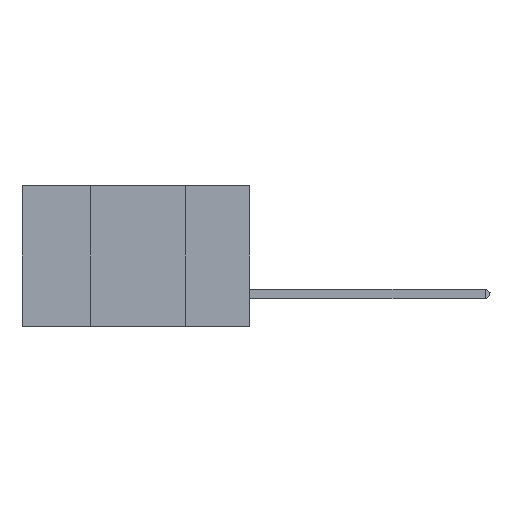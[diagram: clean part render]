
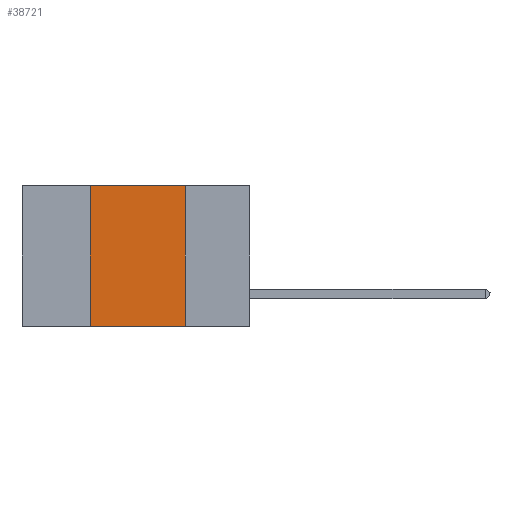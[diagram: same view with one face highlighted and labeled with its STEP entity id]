
A CAD part, left-side view. The second image highlights one B-rep face of the part: STEP entity #38721.
In plain terms, the highlighted planar face has unit normal (-1, 0, 0).
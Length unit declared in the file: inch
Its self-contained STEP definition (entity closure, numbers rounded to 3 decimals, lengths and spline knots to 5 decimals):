
#642 = PLANE ( 'NONE',  #25019 ) ;
#764 = LINE ( 'NONE', #2707, #5825 ) ;
#969 = VERTEX_POINT ( 'NONE', #16987 ) ;
#2707 = CARTESIAN_POINT ( 'NONE',  ( 0., 0.6, -0.37 ) ) ;
#3765 = CARTESIAN_POINT ( 'NONE',  ( 0., 0.6, 0. ) ) ;
#4293 = ORIENTED_EDGE ( 'NONE', *, *, #21761, .F. ) ;
#5825 = VECTOR ( 'NONE', #38327, 39.37008 ) ;
#5847 = CARTESIAN_POINT ( 'NONE',  ( 0., 0.42, 0. ) ) ;
#6810 = VERTEX_POINT ( 'NONE', #34582 ) ;
#7133 = DIRECTION ( 'NONE',  ( 0., 0., -1. ) ) ;
#10416 = VECTOR ( 'NONE', #31794, 39.37008 ) ;
#10791 = DIRECTION ( 'NONE',  ( 1., 0., 0. ) ) ;
#12081 = EDGE_CURVE ( 'NONE', #969, #40265, #764, .T. ) ;
#12092 = ORIENTED_EDGE ( 'NONE', *, *, #32321, .F. ) ;
#13018 = EDGE_LOOP ( 'NONE', ( #12092, #4293, #36905, #40427 ) ) ;
#13136 = LINE ( 'NONE', #5847, #15139 ) ;
#13718 = LINE ( 'NONE', #18140, #22762 ) ;
#15139 = VECTOR ( 'NONE', #28305, 39.37008 ) ;
#15859 = CARTESIAN_POINT ( 'NONE',  ( 0., 0.6, 0. ) ) ;
#16987 = CARTESIAN_POINT ( 'NONE',  ( 0., 0.42, -0.37 ) ) ;
#18140 = CARTESIAN_POINT ( 'NONE',  ( 0., 0.17, 0. ) ) ;
#19389 = VERTEX_POINT ( 'NONE', #21099 ) ;
#19794 = EDGE_CURVE ( 'NONE', #969, #19389, #13136, .T. ) ;
#21099 = CARTESIAN_POINT ( 'NONE',  ( 0., 0.42, 0. ) ) ;
#21761 = EDGE_CURVE ( 'NONE', #19389, #6810, #32947, .T. ) ;
#22762 = VECTOR ( 'NONE', #40653, 39.37008 ) ;
#24966 = CARTESIAN_POINT ( 'NONE',  ( 0., 0.17, -0.37 ) ) ;
#25019 = AXIS2_PLACEMENT_3D ( 'NONE', #3765, #10791, #7133 ) ;
#26207 = FACE_OUTER_BOUND ( 'NONE', #13018, .T. ) ;
#28305 = DIRECTION ( 'NONE',  ( 0., 0., 1. ) ) ;
#31794 = DIRECTION ( 'NONE',  ( 0., -1., 0. ) ) ;
#32321 = EDGE_CURVE ( 'NONE', #6810, #40265, #13718, .T. ) ;
#32947 = LINE ( 'NONE', #15859, #10416 ) ;
#34582 = CARTESIAN_POINT ( 'NONE',  ( 0., 0.17, 0. ) ) ;
#36905 = ORIENTED_EDGE ( 'NONE', *, *, #19794, .F. ) ;
#38327 = DIRECTION ( 'NONE',  ( 0., -1., 0. ) ) ;
#38721 = ADVANCED_FACE ( 'NONE', ( #26207 ), #642, .F. ) ;
#40265 = VERTEX_POINT ( 'NONE', #24966 ) ;
#40427 = ORIENTED_EDGE ( 'NONE', *, *, #12081, .T. ) ;
#40653 = DIRECTION ( 'NONE',  ( 0., 0., -1. ) ) ;
